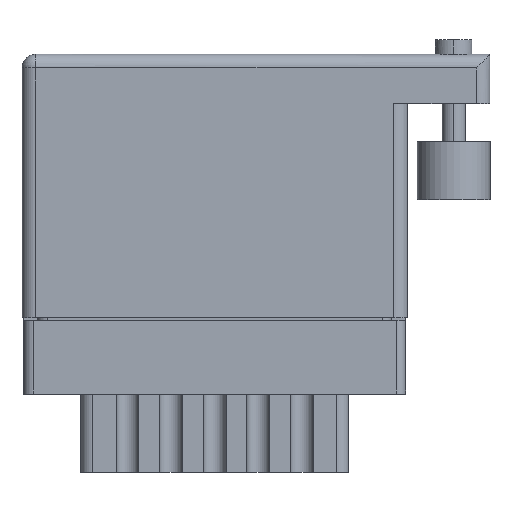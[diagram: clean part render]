
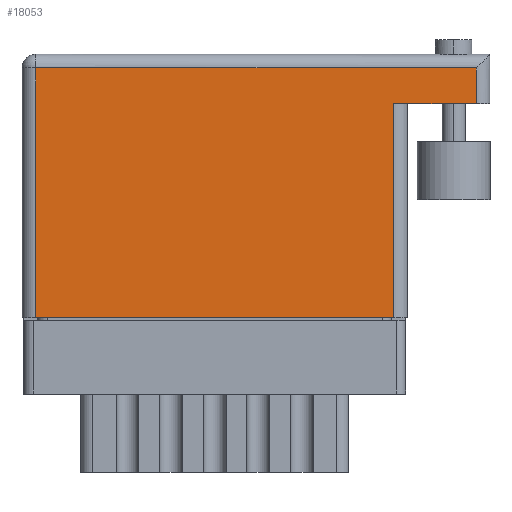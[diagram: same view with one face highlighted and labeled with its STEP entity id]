
A CAD part, front view. The second image highlights one B-rep face of the part: STEP entity #18053.
In plain terms, the highlighted face is planar.
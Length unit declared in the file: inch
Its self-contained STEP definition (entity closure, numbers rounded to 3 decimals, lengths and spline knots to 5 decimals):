
#103 = DIRECTION ( 'NONE',  ( 1., 0., 0. ) ) ;
#1462 = LINE ( 'NONE', #5603, #14021 ) ;
#1583 = VECTOR ( 'NONE', #21705, 39.37008 ) ;
#3316 = AXIS2_PLACEMENT_3D ( 'NONE', #11035, #22188, #4428 ) ;
#3458 = CARTESIAN_POINT ( 'NONE',  ( 1.609, 0.736, 0. ) ) ;
#3629 = EDGE_CURVE ( 'NONE', #8751, #20464, #12533, .T. ) ;
#4428 = DIRECTION ( 'NONE',  ( -1., 0., 0. ) ) ;
#4684 = EDGE_CURVE ( 'NONE', #20464, #16248, #10838, .T. ) ;
#5001 = VECTOR ( 'NONE', #14333, 39.37008 ) ;
#5603 = CARTESIAN_POINT ( 'NONE',  ( 0., 0.859, 0. ) ) ;
#6602 = ORIENTED_EDGE ( 'NONE', *, *, #8473, .T. ) ;
#6851 = VERTEX_POINT ( 'NONE', #21352 ) ;
#7115 = EDGE_CURVE ( 'NONE', #6851, #12450, #19865, .T. ) ;
#7574 = PLANE ( 'NONE',  #3316 ) ;
#7590 = ORIENTED_EDGE ( 'NONE', *, *, #22461, .T. ) ;
#8257 = CARTESIAN_POINT ( 'NONE',  ( 1.562, 0.906, 0. ) ) ;
#8473 = EDGE_CURVE ( 'NONE', #12450, #21934, #1462, .T. ) ;
#8751 = VERTEX_POINT ( 'NONE', #11658 ) ;
#8961 = ORIENTED_EDGE ( 'NONE', *, *, #4684, .T. ) ;
#9089 = DIRECTION ( 'NONE',  ( -1., 0., 0. ) ) ;
#9168 = VECTOR ( 'NONE', #10391, 39.37008 ) ;
#10391 = DIRECTION ( 'NONE',  ( -1., 0., 0. ) ) ;
#10483 = CARTESIAN_POINT ( 'NONE',  ( 0., 0., 0. ) ) ;
#10837 = EDGE_CURVE ( 'NONE', #6851, #16248, #19087, .T. ) ;
#10838 = LINE ( 'NONE', #16377, #1583 ) ;
#11035 = CARTESIAN_POINT ( 'NONE',  ( 0., 0.906, 0. ) ) ;
#11658 = CARTESIAN_POINT ( 'NONE',  ( 0.047, 0., 0. ) ) ;
#12041 = CARTESIAN_POINT ( 'NONE',  ( 1.278, 0., 0. ) ) ;
#12450 = VERTEX_POINT ( 'NONE', #17469 ) ;
#12533 = LINE ( 'NONE', #10483, #13079 ) ;
#13079 = VECTOR ( 'NONE', #103, 39.37008 ) ;
#13611 = CARTESIAN_POINT ( 'NONE',  ( 1.278, 0.736, 0. ) ) ;
#13775 = ORIENTED_EDGE ( 'NONE', *, *, #10837, .F. ) ;
#13967 = DIRECTION ( 'NONE',  ( 0., 1., 0. ) ) ;
#14021 = VECTOR ( 'NONE', #9089, 39.37008 ) ;
#14333 = DIRECTION ( 'NONE',  ( 0., -1., 0. ) ) ;
#15550 = ORIENTED_EDGE ( 'NONE', *, *, #7115, .T. ) ;
#16248 = VERTEX_POINT ( 'NONE', #13611 ) ;
#16377 = CARTESIAN_POINT ( 'NONE',  ( 1.278, 0.736, 0. ) ) ;
#17469 = CARTESIAN_POINT ( 'NONE',  ( 1.562, 0.859, 0. ) ) ;
#18053 = ADVANCED_FACE ( 'NONE', ( #19598 ), #7574, .F. ) ;
#19087 = LINE ( 'NONE', #3458, #9168 ) ;
#19230 = LINE ( 'NONE', #19567, #5001 ) ;
#19567 = CARTESIAN_POINT ( 'NONE',  ( 0.047, 0., 0. ) ) ;
#19598 = FACE_OUTER_BOUND ( 'NONE', #19840, .T. ) ;
#19840 = EDGE_LOOP ( 'NONE', ( #20272, #8961, #13775, #15550, #6602, #7590 ) ) ;
#19865 = LINE ( 'NONE', #8257, #21232 ) ;
#20272 = ORIENTED_EDGE ( 'NONE', *, *, #3629, .T. ) ;
#20464 = VERTEX_POINT ( 'NONE', #12041 ) ;
#21232 = VECTOR ( 'NONE', #13967, 39.37008 ) ;
#21352 = CARTESIAN_POINT ( 'NONE',  ( 1.562, 0.736, 0. ) ) ;
#21581 = CARTESIAN_POINT ( 'NONE',  ( 0.047, 0.859, 0. ) ) ;
#21705 = DIRECTION ( 'NONE',  ( 0., 1., 0. ) ) ;
#21934 = VERTEX_POINT ( 'NONE', #21581 ) ;
#22188 = DIRECTION ( 'NONE',  ( 0., 0., -1. ) ) ;
#22461 = EDGE_CURVE ( 'NONE', #21934, #8751, #19230, .T. ) ;
